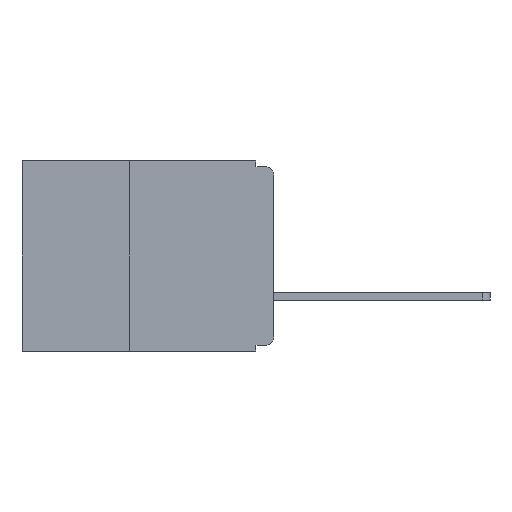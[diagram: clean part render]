
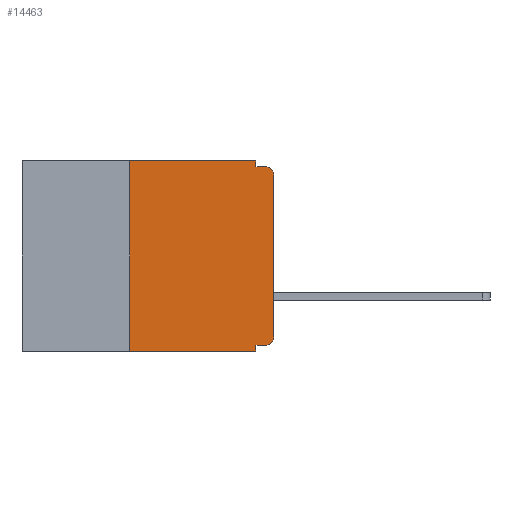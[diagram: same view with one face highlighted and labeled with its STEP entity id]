
A CAD part, left-side view. The second image highlights one B-rep face of the part: STEP entity #14463.
In plain terms, the highlighted planar face has unit normal (-1, 0, 0).
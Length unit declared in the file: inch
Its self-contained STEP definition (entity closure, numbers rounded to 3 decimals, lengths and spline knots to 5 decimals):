
#156 = EDGE_CURVE ( 'NONE', #899, #22756, #19683, .T. ) ;
#829 = EDGE_CURVE ( 'NONE', #22756, #14500, #19340, .T. ) ;
#899 = VERTEX_POINT ( 'NONE', #6674 ) ;
#1331 = LINE ( 'NONE', #11408, #10982 ) ;
#1850 = DIRECTION ( 'NONE',  ( 0., 0., -1. ) ) ;
#2262 = CARTESIAN_POINT ( 'NONE',  ( 0., 0., -0.305 ) ) ;
#2375 = CARTESIAN_POINT ( 'NONE',  ( 0., 0., -0.01 ) ) ;
#3236 = EDGE_CURVE ( 'NONE', #20710, #11445, #11744, .T. ) ;
#3574 = PLANE ( 'NONE',  #12615 ) ;
#3993 = ORIENTED_EDGE ( 'NONE', *, *, #7305, .F. ) ;
#4275 = DIRECTION ( 'NONE',  ( 0., -1., 0. ) ) ;
#4870 = CARTESIAN_POINT ( 'NONE',  ( 0., 0.437, 0. ) ) ;
#5850 = ORIENTED_EDGE ( 'NONE', *, *, #23700, .T. ) ;
#6482 = VECTOR ( 'NONE', #4275, 39.37008 ) ;
#6617 = ORIENTED_EDGE ( 'NONE', *, *, #9397, .F. ) ;
#6674 = CARTESIAN_POINT ( 'NONE',  ( 0., 0.015, -0.32 ) ) ;
#6990 = DIRECTION ( 'NONE',  ( 0., 1., 0. ) ) ;
#7253 = ORIENTED_EDGE ( 'NONE', *, *, #7414, .F. ) ;
#7305 = EDGE_CURVE ( 'NONE', #18997, #21315, #14001, .T. ) ;
#7414 = EDGE_CURVE ( 'NONE', #11034, #23354, #1331, .T. ) ;
#7711 = LINE ( 'NONE', #11636, #12326 ) ;
#8001 = DIRECTION ( 'NONE',  ( 0., 0., 1. ) ) ;
#8173 = CARTESIAN_POINT ( 'NONE',  ( 0., 0.031, -0.01 ) ) ;
#8657 = VERTEX_POINT ( 'NONE', #17320 ) ;
#8697 = CARTESIAN_POINT ( 'NONE',  ( 0., 0., -0.32 ) ) ;
#8703 = DIRECTION ( 'NONE',  ( 0., 0., -1. ) ) ;
#8933 = CARTESIAN_POINT ( 'NONE',  ( 0., 0.031, -0.33 ) ) ;
#9101 = VECTOR ( 'NONE', #8703, 39.37008 ) ;
#9104 = DIRECTION ( 'NONE',  ( 0., 0., 1. ) ) ;
#9219 = ORIENTED_EDGE ( 'NONE', *, *, #14736, .T. ) ;
#9397 = EDGE_CURVE ( 'NONE', #21315, #11034, #24259, .T. ) ;
#9452 = CARTESIAN_POINT ( 'NONE',  ( 0., 0.015, -0.305 ) ) ;
#9474 = CIRCLE ( 'NONE', #24520, 0.015 ) ;
#9680 = DIRECTION ( 'NONE',  ( 0., -1., 0. ) ) ;
#10107 = ORIENTED_EDGE ( 'NONE', *, *, #3236, .T. ) ;
#10323 = CARTESIAN_POINT ( 'NONE',  ( 0., 0.031, 0. ) ) ;
#10982 = VECTOR ( 'NONE', #13332, 39.37008 ) ;
#11025 = CARTESIAN_POINT ( 'NONE',  ( 0., 0.031, -0.32 ) ) ;
#11034 = VERTEX_POINT ( 'NONE', #10323 ) ;
#11210 = FACE_OUTER_BOUND ( 'NONE', #20611, .T. ) ;
#11375 = CARTESIAN_POINT ( 'NONE',  ( 0., 0.437, 0. ) ) ;
#11408 = CARTESIAN_POINT ( 'NONE',  ( 0., 0.031, 0. ) ) ;
#11423 = DIRECTION ( 'NONE',  ( 0., 0., -1. ) ) ;
#11445 = VERTEX_POINT ( 'NONE', #22976 ) ;
#11626 = EDGE_CURVE ( 'NONE', #23354, #8657, #11676, .T. ) ;
#11636 = CARTESIAN_POINT ( 'NONE',  ( 0., 0.437, -0.33 ) ) ;
#11676 = LINE ( 'NONE', #2375, #6482 ) ;
#11744 = LINE ( 'NONE', #18835, #12962 ) ;
#11986 = ORIENTED_EDGE ( 'NONE', *, *, #17913, .T. ) ;
#12023 = ORIENTED_EDGE ( 'NONE', *, *, #156, .F. ) ;
#12125 = AXIS2_PLACEMENT_3D ( 'NONE', #24754, #13397, #1850 ) ;
#12326 = VECTOR ( 'NONE', #9680, 39.37008 ) ;
#12615 = AXIS2_PLACEMENT_3D ( 'NONE', #11375, #24668, #13307 ) ;
#12962 = VECTOR ( 'NONE', #8001, 39.37008 ) ;
#13307 = DIRECTION ( 'NONE',  ( 0., 0., -1. ) ) ;
#13332 = DIRECTION ( 'NONE',  ( 0., 0., -1. ) ) ;
#13397 = DIRECTION ( 'NONE',  ( -1., 0., 0. ) ) ;
#14001 = LINE ( 'NONE', #14941, #24092 ) ;
#14463 = ADVANCED_FACE ( 'NONE', ( #11210 ), #3574, .F. ) ;
#14500 = VERTEX_POINT ( 'NONE', #20976 ) ;
#14736 = EDGE_CURVE ( 'NONE', #11445, #8657, #15393, .T. ) ;
#14941 = CARTESIAN_POINT ( 'NONE',  ( 0., 0.25, -0.33 ) ) ;
#15393 = CIRCLE ( 'NONE', #12125, 0.015 ) ;
#17320 = CARTESIAN_POINT ( 'NONE',  ( 0., 0.015, -0.01 ) ) ;
#17913 = EDGE_CURVE ( 'NONE', #18997, #14500, #7711, .T. ) ;
#18835 = CARTESIAN_POINT ( 'NONE',  ( 0., 0., 0. ) ) ;
#18877 = ORIENTED_EDGE ( 'NONE', *, *, #11626, .F. ) ;
#18967 = ORIENTED_EDGE ( 'NONE', *, *, #829, .F. ) ;
#18997 = VERTEX_POINT ( 'NONE', #20773 ) ;
#19265 = VECTOR ( 'NONE', #22166, 39.37008 ) ;
#19340 = LINE ( 'NONE', #8933, #9101 ) ;
#19683 = LINE ( 'NONE', #8697, #24074 ) ;
#19981 = CARTESIAN_POINT ( 'NONE',  ( 0., 0.25, 0. ) ) ;
#20611 = EDGE_LOOP ( 'NONE', ( #10107, #9219, #18877, #7253, #6617, #3993, #11986, #18967, #12023, #5850 ) ) ;
#20710 = VERTEX_POINT ( 'NONE', #2262 ) ;
#20773 = CARTESIAN_POINT ( 'NONE',  ( 0., 0.25, -0.33 ) ) ;
#20976 = CARTESIAN_POINT ( 'NONE',  ( 0., 0.031, -0.33 ) ) ;
#21315 = VERTEX_POINT ( 'NONE', #19981 ) ;
#22166 = DIRECTION ( 'NONE',  ( 0., -1., 0. ) ) ;
#22756 = VERTEX_POINT ( 'NONE', #11025 ) ;
#22816 = DIRECTION ( 'NONE',  ( -1., 0., 0. ) ) ;
#22976 = CARTESIAN_POINT ( 'NONE',  ( 0., 0., -0.025 ) ) ;
#23354 = VERTEX_POINT ( 'NONE', #8173 ) ;
#23700 = EDGE_CURVE ( 'NONE', #899, #20710, #9474, .T. ) ;
#24074 = VECTOR ( 'NONE', #6990, 39.37008 ) ;
#24092 = VECTOR ( 'NONE', #9104, 39.37008 ) ;
#24259 = LINE ( 'NONE', #4870, #19265 ) ;
#24520 = AXIS2_PLACEMENT_3D ( 'NONE', #9452, #22816, #11423 ) ;
#24668 = DIRECTION ( 'NONE',  ( 1., 0., 0. ) ) ;
#24754 = CARTESIAN_POINT ( 'NONE',  ( 0., 0.015, -0.025 ) ) ;
